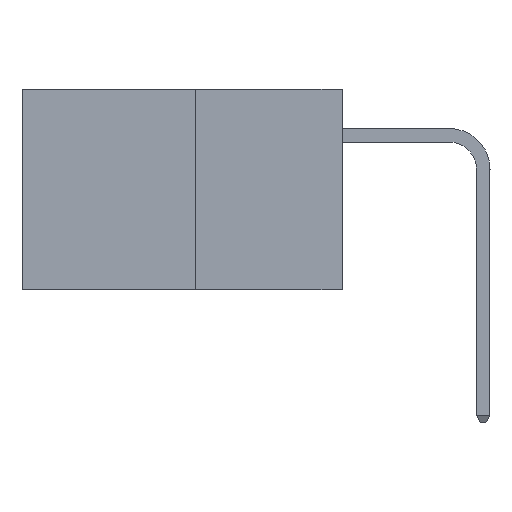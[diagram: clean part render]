
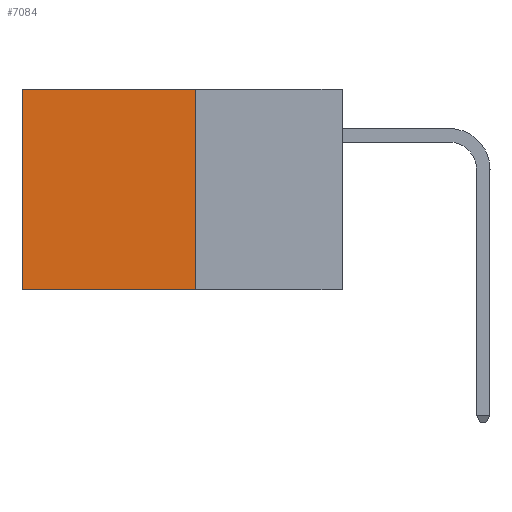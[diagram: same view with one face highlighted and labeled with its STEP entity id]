
A CAD part, left-side view. The second image highlights one B-rep face of the part: STEP entity #7084.
In plain terms, the highlighted planar face has unit normal (-1, 0, 0).
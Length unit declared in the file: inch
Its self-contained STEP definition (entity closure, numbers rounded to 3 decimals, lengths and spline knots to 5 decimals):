
#202 = CARTESIAN_POINT ( 'NONE',  ( 0.277, 0.27, -0.37 ) ) ;
#509 = AXIS2_PLACEMENT_3D ( 'NONE', #25554, #27626, #15015 ) ;
#1550 = VECTOR ( 'NONE', #21725, 39.37008 ) ;
#1715 = VERTEX_POINT ( 'NONE', #9537 ) ;
#2872 = LINE ( 'NONE', #24357, #19403 ) ;
#3413 = LINE ( 'NONE', #25443, #24879 ) ;
#6561 = CARTESIAN_POINT ( 'NONE',  ( 0.277, 0.59, -0.37 ) ) ;
#6856 = LINE ( 'NONE', #25788, #16964 ) ;
#7084 = ADVANCED_FACE ( 'NONE', ( #13689 ), #10716, .F. ) ;
#8819 = ORIENTED_EDGE ( 'NONE', *, *, #15116, .F. ) ;
#9537 = CARTESIAN_POINT ( 'NONE',  ( 0.277, 0.27, -0.37 ) ) ;
#10305 = VERTEX_POINT ( 'NONE', #20979 ) ;
#10716 = PLANE ( 'NONE',  #509 ) ;
#11061 = DIRECTION ( 'NONE',  ( 0., 0., -1. ) ) ;
#11732 = DIRECTION ( 'NONE',  ( 0., 0., -1. ) ) ;
#13689 = FACE_OUTER_BOUND ( 'NONE', #26009, .T. ) ;
#13827 = LINE ( 'NONE', #202, #1550 ) ;
#15015 = DIRECTION ( 'NONE',  ( 0., 0., -1. ) ) ;
#15116 = EDGE_CURVE ( 'NONE', #10305, #1715, #6856, .T. ) ;
#16964 = VECTOR ( 'NONE', #11061, 39.37008 ) ;
#17968 = VERTEX_POINT ( 'NONE', #6561 ) ;
#18935 = EDGE_CURVE ( 'NONE', #19326, #17968, #2872, .T. ) ;
#19326 = VERTEX_POINT ( 'NONE', #27698 ) ;
#19403 = VECTOR ( 'NONE', #11732, 39.37008 ) ;
#20979 = CARTESIAN_POINT ( 'NONE',  ( 0.277, 0.27, 0. ) ) ;
#21094 = EDGE_CURVE ( 'NONE', #10305, #19326, #3413, .T. ) ;
#21519 = ORIENTED_EDGE ( 'NONE', *, *, #23650, .F. ) ;
#21725 = DIRECTION ( 'NONE',  ( 0., 1., 0. ) ) ;
#22233 = ORIENTED_EDGE ( 'NONE', *, *, #21094, .T. ) ;
#23650 = EDGE_CURVE ( 'NONE', #1715, #17968, #13827, .T. ) ;
#23970 = ORIENTED_EDGE ( 'NONE', *, *, #18935, .T. ) ;
#24357 = CARTESIAN_POINT ( 'NONE',  ( 0.277, 0.59, -0.37 ) ) ;
#24879 = VECTOR ( 'NONE', #27530, 39.37008 ) ;
#25443 = CARTESIAN_POINT ( 'NONE',  ( 0.277, 0.27, 0. ) ) ;
#25554 = CARTESIAN_POINT ( 'NONE',  ( 0.277, 0.27, -0.37 ) ) ;
#25788 = CARTESIAN_POINT ( 'NONE',  ( 0.277, 0.27, -0.37 ) ) ;
#26009 = EDGE_LOOP ( 'NONE', ( #23970, #21519, #8819, #22233 ) ) ;
#27530 = DIRECTION ( 'NONE',  ( 0., 1., 0. ) ) ;
#27626 = DIRECTION ( 'NONE',  ( 1., 0., 0. ) ) ;
#27698 = CARTESIAN_POINT ( 'NONE',  ( 0.277, 0.59, 0. ) ) ;
